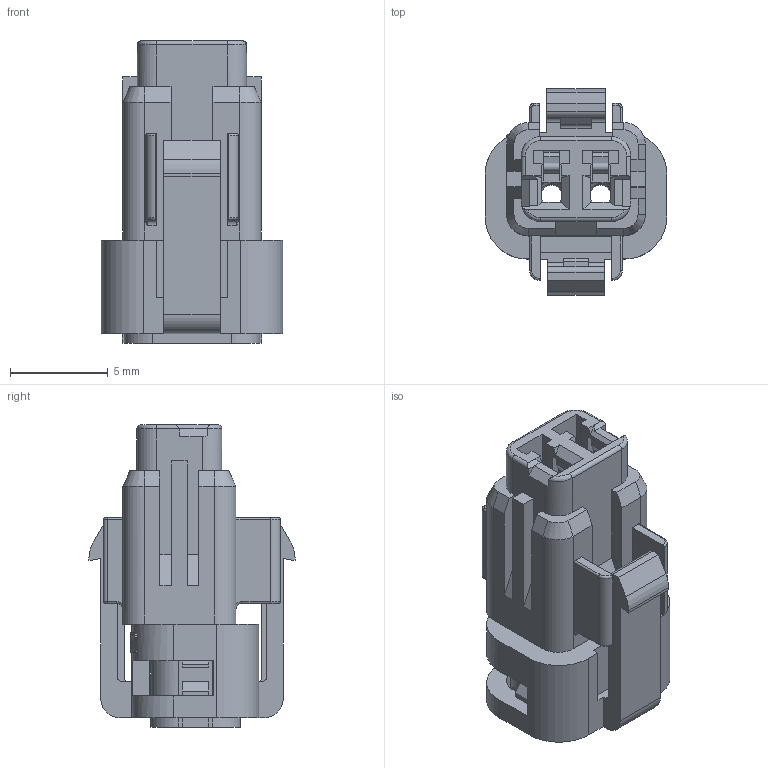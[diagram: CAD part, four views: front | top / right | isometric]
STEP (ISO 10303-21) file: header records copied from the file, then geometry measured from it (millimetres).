
FILE_DESCRIPTION (( 'STEP AP203' ), '1' );
FILE_NAME ('560-002-000-410.STEP', '2020-07-24T15:19:30', ( '' ), ( '' ), 'SwSTEP 2.0', 'SolidWorks 2020', '' );
FILE_SCHEMA (( 'CONFIG_CONTROL_DESIGN' ));
Length unit declared in the file: millimetre
Products named in the file (5): 560-002-000-410; FEMALE-HOUSING-2POS_BLUE; INSULATOR-2POS-1; REAR-GASKET-2POS_YELLOW
Assembly tree (4 placements, depth 3):
  560-002-000-410
    560-002-000-410
      FEMALE-HOUSING-2POS_BLUE
      INSULATOR-2POS-1
      REAR-GASKET-2POS_YELLOW
Bounding box: 9.3 x 10.55 x 15.48 mm (x, y, z)
Volume: 544.9 mm3; surface area: 1381 mm2
Topology: 3 solids, 3 shells, 656 faces, 1754 edges, 1108 vertices
Faces by surface type: plane 401, cylinder 139, torus 64, cone 52
Entity records: 21002 total; most frequent: CARTESIAN_POINT 4111, ORIENTED_EDGE 3508, DIRECTION 3325, EDGE_CURVE 1754, LINE 1217, VECTOR 1217, VERTEX_POINT 1108, AXIS2_PLACEMENT_3D 1054
